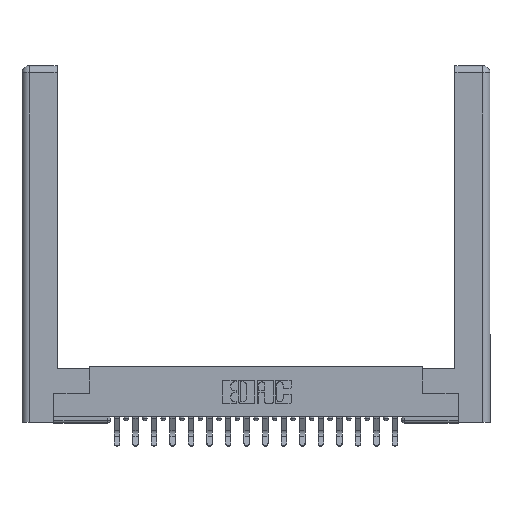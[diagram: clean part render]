
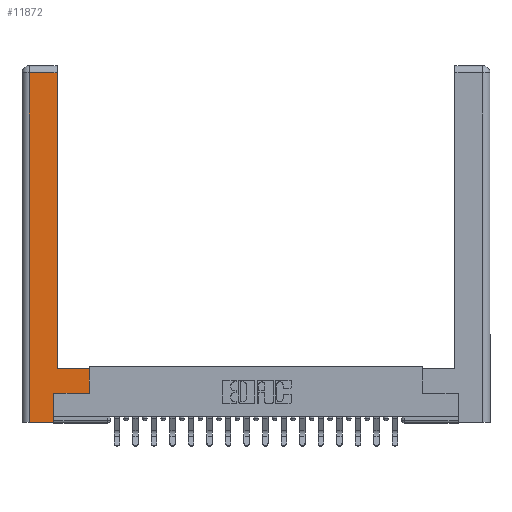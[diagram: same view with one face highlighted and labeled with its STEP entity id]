
A CAD part, top view. The second image highlights one B-rep face of the part: STEP entity #11872.
In plain terms, the highlighted planar face has unit normal (0, 0, 1).
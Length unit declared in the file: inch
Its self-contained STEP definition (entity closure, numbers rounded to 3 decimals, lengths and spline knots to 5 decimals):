
#203 = CARTESIAN_POINT ( 'NONE',  ( 0.0615, 2.94, 0. ) ) ;
#266 = ORIENTED_EDGE ( 'NONE', *, *, #17762, .T. ) ;
#353 = ORIENTED_EDGE ( 'NONE', *, *, #12894, .T. ) ;
#508 = CARTESIAN_POINT ( 'NONE',  ( 0.0615, 2.94, 0. ) ) ;
#581 = DIRECTION ( 'NONE',  ( 0., 1., 0. ) ) ;
#601 = ORIENTED_EDGE ( 'NONE', *, *, #3573, .T. ) ;
#986 = EDGE_CURVE ( 'NONE', #6223, #2371, #3539, .T. ) ;
#1087 = DIRECTION ( 'NONE',  ( 1., 0., 0. ) ) ;
#1145 = DIRECTION ( 'NONE',  ( 0., -1., 0. ) ) ;
#2084 = CARTESIAN_POINT ( 'NONE',  ( 0.295, 2.94, 0. ) ) ;
#2349 = VECTOR ( 'NONE', #16038, 39.37008 ) ;
#2371 = VERTEX_POINT ( 'NONE', #7299 ) ;
#2459 = VECTOR ( 'NONE', #6803, 39.37008 ) ;
#2632 = ORIENTED_EDGE ( 'NONE', *, *, #17490, .T. ) ;
#2736 = CARTESIAN_POINT ( 'NONE',  ( 0.265, 0., 0. ) ) ;
#2781 = ORIENTED_EDGE ( 'NONE', *, *, #5977, .T. ) ;
#3539 = LINE ( 'NONE', #2736, #14253 ) ;
#3573 = EDGE_CURVE ( 'NONE', #10331, #4062, #4725, .T. ) ;
#3757 = DIRECTION ( 'NONE',  ( 0., 0., -1. ) ) ;
#3833 = ORIENTED_EDGE ( 'NONE', *, *, #986, .T. ) ;
#4062 = VERTEX_POINT ( 'NONE', #2084 ) ;
#4165 = LINE ( 'NONE', #8962, #18788 ) ;
#4472 = LINE ( 'NONE', #508, #17386 ) ;
#4501 = CARTESIAN_POINT ( 'NONE',  ( 0.565, 0.245, 0. ) ) ;
#4725 = LINE ( 'NONE', #13130, #8136 ) ;
#4813 = VERTEX_POINT ( 'NONE', #203 ) ;
#4980 = VERTEX_POINT ( 'NONE', #5051 ) ;
#5051 = CARTESIAN_POINT ( 'NONE',  ( 0.265, 0.245, 0. ) ) ;
#5553 = LINE ( 'NONE', #18402, #7014 ) ;
#5634 = VERTEX_POINT ( 'NONE', #9323 ) ;
#5933 = ORIENTED_EDGE ( 'NONE', *, *, #20018, .T. ) ;
#5977 = EDGE_CURVE ( 'NONE', #4980, #17315, #4165, .T. ) ;
#6223 = VERTEX_POINT ( 'NONE', #17051 ) ;
#6803 = DIRECTION ( 'NONE',  ( -1., 0., 0. ) ) ;
#7014 = VECTOR ( 'NONE', #1145, 39.37008 ) ;
#7299 = CARTESIAN_POINT ( 'NONE',  ( 0.265, 0., 0. ) ) ;
#7625 = CARTESIAN_POINT ( 'NONE',  ( 0.265, 0.245, 0. ) ) ;
#8136 = VECTOR ( 'NONE', #581, 39.37008 ) ;
#8937 = DIRECTION ( 'NONE',  ( 1., 0., 0. ) ) ;
#8962 = CARTESIAN_POINT ( 'NONE',  ( 0.565, 0.245, 0. ) ) ;
#9057 = FACE_OUTER_BOUND ( 'NONE', #12945, .T. ) ;
#9087 = CARTESIAN_POINT ( 'NONE',  ( 0.295, 0.45, 0. ) ) ;
#9323 = CARTESIAN_POINT ( 'NONE',  ( 0.565, 0.45, 0. ) ) ;
#10331 = VERTEX_POINT ( 'NONE', #9087 ) ;
#10750 = EDGE_CURVE ( 'NONE', #4062, #4813, #4472, .T. ) ;
#11169 = CARTESIAN_POINT ( 'NONE',  ( 0.295, 0.45, 0. ) ) ;
#11349 = DIRECTION ( 'NONE',  ( -1., 0., 0. ) ) ;
#11872 = ADVANCED_FACE ( 'NONE', ( #9057 ), #16110, .F. ) ;
#12050 = LINE ( 'NONE', #12992, #2349 ) ;
#12894 = EDGE_CURVE ( 'NONE', #2371, #4980, #15378, .T. ) ;
#12945 = EDGE_LOOP ( 'NONE', ( #601, #17967, #266, #3833, #353, #2781, #5933, #2632 ) ) ;
#12992 = CARTESIAN_POINT ( 'NONE',  ( 0.565, 0.45, 0. ) ) ;
#13000 = CARTESIAN_POINT ( 'NONE',  ( 0., 0., 0. ) ) ;
#13130 = CARTESIAN_POINT ( 'NONE',  ( 0.295, 3., 0. ) ) ;
#14253 = VECTOR ( 'NONE', #8937, 39.37008 ) ;
#14580 = AXIS2_PLACEMENT_3D ( 'NONE', #13000, #3757, #19319 ) ;
#15378 = LINE ( 'NONE', #7625, #19080 ) ;
#16038 = DIRECTION ( 'NONE',  ( 0., 1., 0. ) ) ;
#16042 = LINE ( 'NONE', #11169, #2459 ) ;
#16110 = PLANE ( 'NONE',  #14580 ) ;
#17051 = CARTESIAN_POINT ( 'NONE',  ( 0.0615, 0., 0. ) ) ;
#17315 = VERTEX_POINT ( 'NONE', #4501 ) ;
#17386 = VECTOR ( 'NONE', #11349, 39.37008 ) ;
#17490 = EDGE_CURVE ( 'NONE', #5634, #10331, #16042, .T. ) ;
#17762 = EDGE_CURVE ( 'NONE', #4813, #6223, #5553, .T. ) ;
#17967 = ORIENTED_EDGE ( 'NONE', *, *, #10750, .T. ) ;
#18402 = CARTESIAN_POINT ( 'NONE',  ( 0.0615, 0., 0. ) ) ;
#18554 = DIRECTION ( 'NONE',  ( 0., 1., 0. ) ) ;
#18788 = VECTOR ( 'NONE', #1087, 39.37008 ) ;
#19080 = VECTOR ( 'NONE', #18554, 39.37008 ) ;
#19319 = DIRECTION ( 'NONE',  ( -1., 0., 0. ) ) ;
#20018 = EDGE_CURVE ( 'NONE', #17315, #5634, #12050, .T. ) ;
